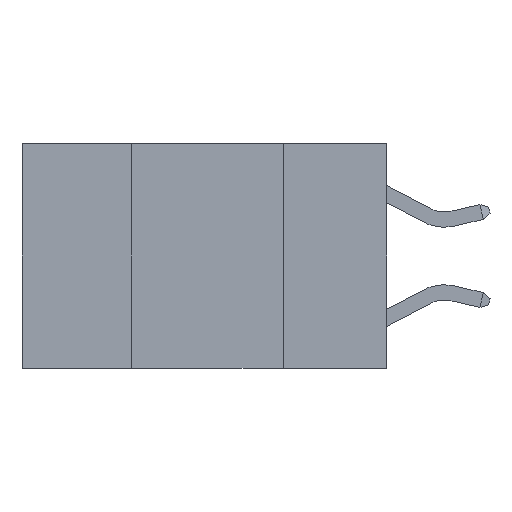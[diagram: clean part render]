
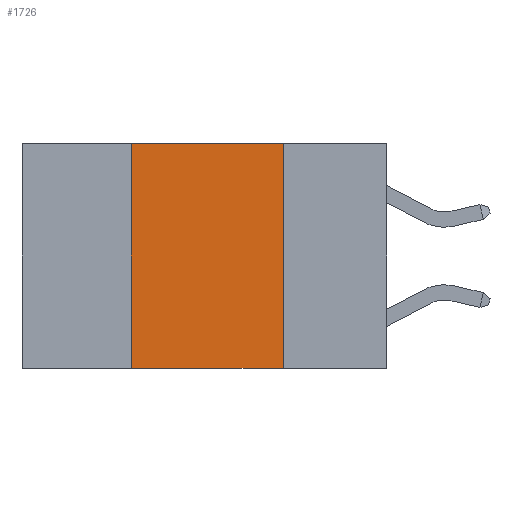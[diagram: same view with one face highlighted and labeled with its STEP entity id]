
A CAD part, left-side view. The second image highlights one B-rep face of the part: STEP entity #1726.
In plain terms, the highlighted planar face has unit normal (-1, 0, 0).
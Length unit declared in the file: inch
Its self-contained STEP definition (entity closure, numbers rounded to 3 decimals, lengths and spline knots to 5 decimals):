
#59 = VERTEX_POINT ( 'NONE', #12373 ) ;
#239 = LINE ( 'NONE', #6218, #2558 ) ;
#766 = CARTESIAN_POINT ( 'NONE',  ( 0., 0.17, -0.37 ) ) ;
#1149 = DIRECTION ( 'NONE',  ( 0., -1., 0. ) ) ;
#1488 = CARTESIAN_POINT ( 'NONE',  ( 0., 0.6, -0.37 ) ) ;
#1574 = ORIENTED_EDGE ( 'NONE', *, *, #8853, .F. ) ;
#1658 = LINE ( 'NONE', #8021, #6607 ) ;
#1726 = ADVANCED_FACE ( 'NONE', ( #2401 ), #7521, .F. ) ;
#1751 = VECTOR ( 'NONE', #8151, 39.37008 ) ;
#1872 = DIRECTION ( 'NONE',  ( 1., 0., 0. ) ) ;
#1992 = ORIENTED_EDGE ( 'NONE', *, *, #10878, .F. ) ;
#2218 = CARTESIAN_POINT ( 'NONE',  ( 0., 0.6, 0. ) ) ;
#2401 = FACE_OUTER_BOUND ( 'NONE', #5877, .T. ) ;
#2558 = VECTOR ( 'NONE', #11117, 39.37008 ) ;
#2559 = ORIENTED_EDGE ( 'NONE', *, *, #7559, .F. ) ;
#2680 = ORIENTED_EDGE ( 'NONE', *, *, #7807, .T. ) ;
#3237 = VERTEX_POINT ( 'NONE', #12533 ) ;
#3976 = VERTEX_POINT ( 'NONE', #766 ) ;
#4356 = AXIS2_PLACEMENT_3D ( 'NONE', #2218, #1872, #7581 ) ;
#5877 = EDGE_LOOP ( 'NONE', ( #1574, #2559, #1992, #2680 ) ) ;
#6218 = CARTESIAN_POINT ( 'NONE',  ( 0., 0.17, 0. ) ) ;
#6607 = VECTOR ( 'NONE', #1149, 39.37008 ) ;
#7068 = LINE ( 'NONE', #1488, #11691 ) ;
#7124 = VERTEX_POINT ( 'NONE', #7363 ) ;
#7159 = CARTESIAN_POINT ( 'NONE',  ( 0., 0.42, 0. ) ) ;
#7363 = CARTESIAN_POINT ( 'NONE',  ( 0., 0.17, 0. ) ) ;
#7521 = PLANE ( 'NONE',  #4356 ) ;
#7559 = EDGE_CURVE ( 'NONE', #59, #7124, #1658, .T. ) ;
#7581 = DIRECTION ( 'NONE',  ( 0., 0., -1. ) ) ;
#7807 = EDGE_CURVE ( 'NONE', #3237, #3976, #7068, .T. ) ;
#8021 = CARTESIAN_POINT ( 'NONE',  ( 0., 0.6, 0. ) ) ;
#8151 = DIRECTION ( 'NONE',  ( 0., 0., 1. ) ) ;
#8853 = EDGE_CURVE ( 'NONE', #7124, #3976, #239, .T. ) ;
#9390 = DIRECTION ( 'NONE',  ( 0., -1., 0. ) ) ;
#10878 = EDGE_CURVE ( 'NONE', #3237, #59, #12236, .T. ) ;
#11117 = DIRECTION ( 'NONE',  ( 0., 0., -1. ) ) ;
#11691 = VECTOR ( 'NONE', #9390, 39.37008 ) ;
#12236 = LINE ( 'NONE', #7159, #1751 ) ;
#12373 = CARTESIAN_POINT ( 'NONE',  ( 0., 0.42, 0. ) ) ;
#12533 = CARTESIAN_POINT ( 'NONE',  ( 0., 0.42, -0.37 ) ) ;
